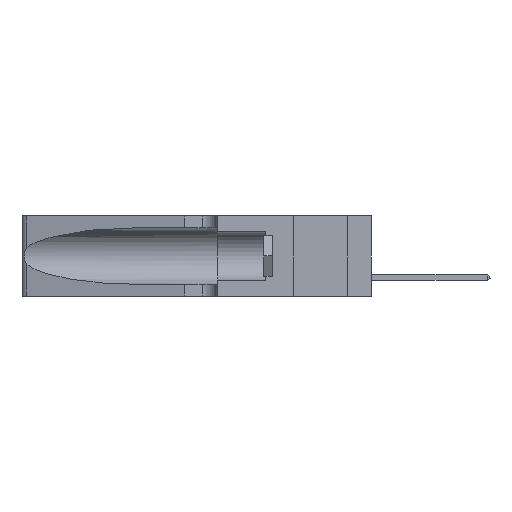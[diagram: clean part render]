
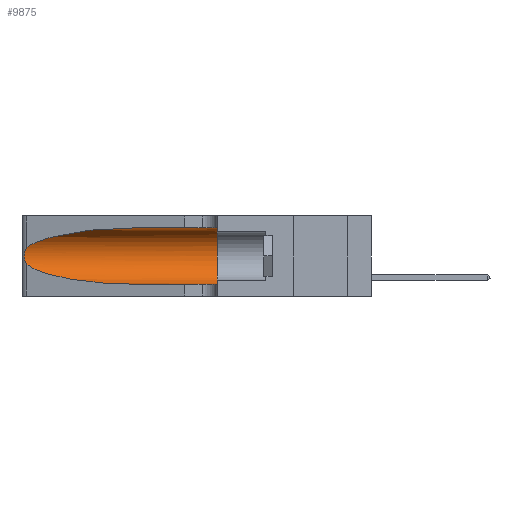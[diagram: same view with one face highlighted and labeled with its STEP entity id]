
A CAD part, left-side view. The second image highlights one B-rep face of the part: STEP entity #9875.
In plain terms, the highlighted cylindrical face has radius 3.308 mm (diameter 6.617 mm), a partial arc.
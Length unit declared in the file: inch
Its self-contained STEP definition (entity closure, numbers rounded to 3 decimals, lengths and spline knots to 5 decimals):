
#472 = CARTESIAN_POINT ( 'NONE',  ( 0.1305, 0.35, 0.05475 ) ) ;
#767 = FACE_OUTER_BOUND ( 'NONE', #23333, .T. ) ;
#3520 = EDGE_CURVE ( 'NONE', #31884, #22844, #6249, .T. ) ;
#3557 = CARTESIAN_POINT ( 'NONE',  ( 0.26018, 1.23835, 0.19895 ) ) ;
#4036 = LINE ( 'NONE', #5983, #30842 ) ;
#4738 = EDGE_CURVE ( 'NONE', #30986, #23327, #4036, .T. ) ;
#5946 = DIRECTION ( 'NONE',  ( 0., -1., 0. ) ) ;
#5983 = CARTESIAN_POINT ( 'NONE',  ( 0.1305, 1.61858, 0.31525 ) ) ;
#6249 = LINE ( 'NONE', #18782, #11902 ) ;
#6380 = CARTESIAN_POINT ( 'NONE',  ( 0.1305, 1.61858, 0.185 ) ) ;
#6856 = CARTESIAN_POINT ( 'NONE',  ( 0.25555, 1.22994, 0.2215 ) ) ;
#7051 = CARTESIAN_POINT ( 'NONE',  ( 0.2373, 1.15595, 0.28018 ) ) ;
#7428 = CARTESIAN_POINT ( 'NONE',  ( 0.25787, 1.23484, 0.2124 ) ) ;
#8370 = ORIENTED_EDGE ( 'NONE', *, *, #4738, .F. ) ;
#9040 = EDGE_CURVE ( 'NONE', #10047, #32097, #20530, .T. ) ;
#9875 = ADVANCED_FACE ( 'NONE', ( #767 ), #21411, .F. ) ;
#10047 = VERTEX_POINT ( 'NONE', #22039 ) ;
#10389 = CARTESIAN_POINT ( 'NONE',  ( 0.1305, 0.72297, 0.05475 ) ) ;
#10594 = CARTESIAN_POINT ( 'NONE',  ( 0.25854, 1.2359, 0.20912 ) ) ;
#11487 = EDGE_CURVE ( 'NONE', #32097, #31884, #40280, .T. ) ;
#11902 = VECTOR ( 'NONE', #5946, 39.37008 ) ;
#13610 = CARTESIAN_POINT ( 'NONE',  ( 0.25555, 1.22993, 0.14849 ) ) ;
#13758 = CARTESIAN_POINT ( 'NONE',  ( 0.25487, 1.22718, 0.22369 ) ) ;
#15582 = EDGE_CURVE ( 'NONE', #30986, #10047, #42158, .T. ) ;
#16462 = CARTESIAN_POINT ( 'NONE',  ( 0.1305, 0.72297, 0.31525 ) ) ;
#16677 = CARTESIAN_POINT ( 'NONE',  ( 0.26017, 1.23833, 0.17102 ) ) ;
#17249 = CARTESIAN_POINT ( 'NONE',  ( 0.25856, 1.23593, 0.16098 ) ) ;
#17282 = CARTESIAN_POINT ( 'NONE',  ( 0.1305, 0.72297, 0.31525 ) ) ;
#17316 = EDGE_CURVE ( 'NONE', #23327, #22844, #32057, .T. ) ;
#18344 = CARTESIAN_POINT ( 'NONE',  ( 0.25487, 1.22718, 0.14631 ) ) ;
#18782 = CARTESIAN_POINT ( 'NONE',  ( 0.1305, 1.61858, 0.05475 ) ) ;
#19274 = CARTESIAN_POINT ( 'NONE',  ( 0.1305, 0.35, 0.31525 ) ) ;
#19581 = ORIENTED_EDGE ( 'NONE', *, *, #9040, .T. ) ;
#20250 = CARTESIAN_POINT ( 'NONE',  ( 0.25487, 1.22718, 0.14631 ) ) ;
#20530 = B_SPLINE_CURVE_WITH_KNOTS ( 'NONE', 3,
 ( #13758, #6856, #36631, #7428, #10594, #3557, #39664, #23581, #16677, #17249, #33627, #39797, #13610, #20250 ),
 .UNSPECIFIED., .F., .F.,
 ( 4, 2, 2, 2, 2, 2, 4 ),
 ( 0., 0.00027, 0.00053, 0.00107, 0.0016, 0.00187, 0.00214 ),
 .UNSPECIFIED. ) ;
#20824 = ORIENTED_EDGE ( 'NONE', *, *, #17316, .F. ) ;
#21345 = CARTESIAN_POINT ( 'NONE',  ( 0.2373, 1.15595, 0.08982 ) ) ;
#21411 = CYLINDRICAL_SURFACE ( 'NONE', #22329, 0.13025 ) ;
#22039 = CARTESIAN_POINT ( 'NONE',  ( 0.25487, 1.22718, 0.22369 ) ) ;
#22329 = AXIS2_PLACEMENT_3D ( 'NONE', #6380, #42342, #29594 ) ;
#22689 = DIRECTION ( 'NONE',  ( 0., -1., 0. ) ) ;
#22844 = VERTEX_POINT ( 'NONE', #472 ) ;
#22940 = ORIENTED_EDGE ( 'NONE', *, *, #3520, .T. ) ;
#23190 = CARTESIAN_POINT ( 'NONE',  ( 0.18966, 0.96281, 0.31525 ) ) ;
#23327 = VERTEX_POINT ( 'NONE', #19274 ) ;
#23333 = EDGE_LOOP ( 'NONE', ( #28731, #19581, #32292, #22940, #20824, #8370 ) ) ;
#23581 = CARTESIAN_POINT ( 'NONE',  ( 0.26075, 1.23896, 0.178 ) ) ;
#26144 = CARTESIAN_POINT ( 'NONE',  ( 0.1305, 0.35, 0.185 ) ) ;
#28731 = ORIENTED_EDGE ( 'NONE', *, *, #15582, .T. ) ;
#29027 = DIRECTION ( 'NONE',  ( 0., 0., 1. ) ) ;
#29594 = DIRECTION ( 'NONE',  ( 0., 0., -1. ) ) ;
#30534 = CARTESIAN_POINT ( 'NONE',  ( 0.25487, 1.22718, 0.14631 ) ) ;
#30842 = VECTOR ( 'NONE', #22689, 39.37008 ) ;
#30986 = VERTEX_POINT ( 'NONE', #17282 ) ;
#31311 = CARTESIAN_POINT ( 'NONE',  ( 0.18966, 0.96281, 0.05475 ) ) ;
#31884 = VERTEX_POINT ( 'NONE', #10389 ) ;
#32057 = CIRCLE ( 'NONE', #33216, 0.13025 ) ;
#32097 = VERTEX_POINT ( 'NONE', #30534 ) ;
#32292 = ORIENTED_EDGE ( 'NONE', *, *, #11487, .T. ) ;
#32732 = DIRECTION ( 'NONE',  ( 0., 1., 0. ) ) ;
#33216 = AXIS2_PLACEMENT_3D ( 'NONE', #26144, #32732, #29027 ) ;
#33388 = CARTESIAN_POINT ( 'NONE',  ( 0.25487, 1.22718, 0.22369 ) ) ;
#33627 = CARTESIAN_POINT ( 'NONE',  ( 0.25789, 1.23486, 0.15765 ) ) ;
#36631 = CARTESIAN_POINT ( 'NONE',  ( 0.25639, 1.23184, 0.21858 ) ) ;
#39664 = CARTESIAN_POINT ( 'NONE',  ( 0.26075, 1.23896, 0.19203 ) ) ;
#39797 = CARTESIAN_POINT ( 'NONE',  ( 0.25639, 1.23186, 0.15144 ) ) ;
#40280 =( BOUNDED_CURVE ( )  B_SPLINE_CURVE ( 3, ( #18344, #21345, #31311, #41316 ),
 .UNSPECIFIED., .F., .T. ) 
 B_SPLINE_CURVE_WITH_KNOTS ( ( 4, 4 ),
 ( 3.44316, 4.71239 ),
 .UNSPECIFIED. ) 
 CURVE ( )  GEOMETRIC_REPRESENTATION_ITEM ( )  RATIONAL_B_SPLINE_CURVE ( ( 1., 0.87, 0.87, 1. ) ) 
 REPRESENTATION_ITEM ( '' )  );
#41316 = CARTESIAN_POINT ( 'NONE',  ( 0.1305, 0.72297, 0.05475 ) ) ;
#42158 =( BOUNDED_CURVE ( )  B_SPLINE_CURVE ( 3, ( #16462, #23190, #7051, #33388 ),
 .UNSPECIFIED., .F., .F. ) 
 B_SPLINE_CURVE_WITH_KNOTS ( ( 4, 4 ),
 ( 1.5708, 2.84003 ),
 .UNSPECIFIED. ) 
 CURVE ( )  GEOMETRIC_REPRESENTATION_ITEM ( )  RATIONAL_B_SPLINE_CURVE ( ( 1., 0.87, 0.87, 1. ) ) 
 REPRESENTATION_ITEM ( '' )  );
#42342 = DIRECTION ( 'NONE',  ( 0., -1., 0. ) ) ;
